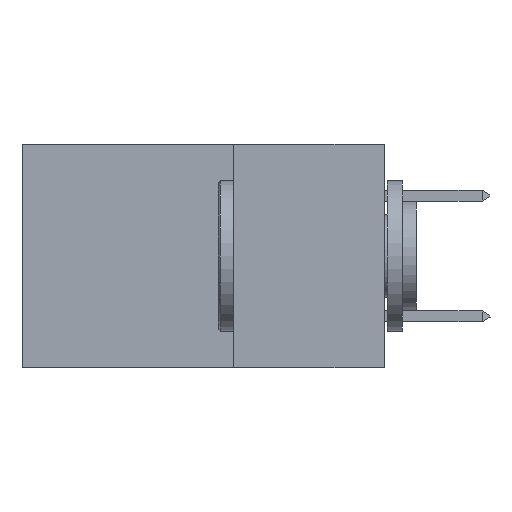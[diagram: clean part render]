
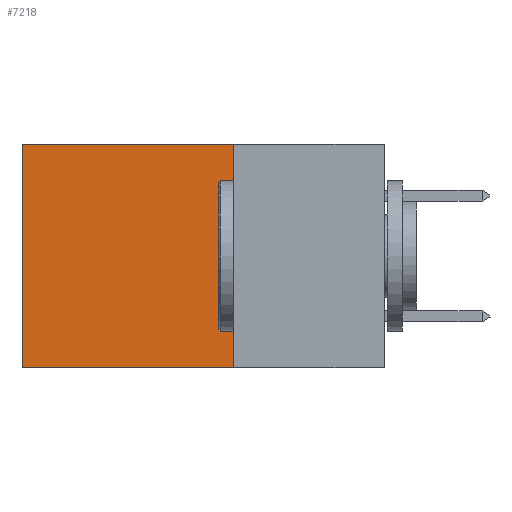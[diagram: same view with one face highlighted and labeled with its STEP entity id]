
A CAD part, left-side view. The second image highlights one B-rep face of the part: STEP entity #7218.
In plain terms, the highlighted planar face has unit normal (-1, 0, 0).
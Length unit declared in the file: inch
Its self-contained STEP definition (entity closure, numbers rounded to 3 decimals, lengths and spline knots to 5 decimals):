
#7 = FACE_OUTER_BOUND ( 'NONE', #13124, .T. ) ;
#71 = DIRECTION ( 'NONE',  ( 1., 0., 0. ) ) ;
#235 = CARTESIAN_POINT ( 'NONE',  ( 0.2875, 0.25, 0. ) ) ;
#415 = VECTOR ( 'NONE', #11790, 39.37008 ) ;
#1043 = ORIENTED_EDGE ( 'NONE', *, *, #7976, .F. ) ;
#1369 = EDGE_CURVE ( 'NONE', #7098, #1430, #12800, .T. ) ;
#1430 = VERTEX_POINT ( 'NONE', #6692 ) ;
#2300 = LINE ( 'NONE', #13733, #8791 ) ;
#2310 = VECTOR ( 'NONE', #9135, 39.37008 ) ;
#2949 = CARTESIAN_POINT ( 'NONE',  ( 0.2875, 0.25, -0.37 ) ) ;
#3578 = DIRECTION ( 'NONE',  ( 0., 1., 0. ) ) ;
#3686 = PLANE ( 'NONE',  #6498 ) ;
#3826 = CARTESIAN_POINT ( 'NONE',  ( 0.2875, 0.25, 0. ) ) ;
#4087 = LINE ( 'NONE', #6836, #2310 ) ;
#4740 = DIRECTION ( 'NONE',  ( 0., 1., 0. ) ) ;
#6018 = EDGE_CURVE ( 'NONE', #7098, #9518, #9941, .T. ) ;
#6498 = AXIS2_PLACEMENT_3D ( 'NONE', #235, #71, #8244 ) ;
#6692 = CARTESIAN_POINT ( 'NONE',  ( 0.2875, 0.6, 0. ) ) ;
#6818 = VERTEX_POINT ( 'NONE', #8140 ) ;
#6836 = CARTESIAN_POINT ( 'NONE',  ( 0.2875, 0.6, 0. ) ) ;
#7098 = VERTEX_POINT ( 'NONE', #10481 ) ;
#7218 = ADVANCED_FACE ( 'NONE', ( #7 ), #3686, .F. ) ;
#7976 = EDGE_CURVE ( 'NONE', #9518, #6818, #2300, .T. ) ;
#8140 = CARTESIAN_POINT ( 'NONE',  ( 0.2875, 0.6, -0.37 ) ) ;
#8244 = DIRECTION ( 'NONE',  ( 0., 0., -1. ) ) ;
#8563 = ORIENTED_EDGE ( 'NONE', *, *, #6018, .F. ) ;
#8639 = ORIENTED_EDGE ( 'NONE', *, *, #11719, .T. ) ;
#8791 = VECTOR ( 'NONE', #4740, 39.37008 ) ;
#9135 = DIRECTION ( 'NONE',  ( 0., 0., -1. ) ) ;
#9518 = VERTEX_POINT ( 'NONE', #2949 ) ;
#9557 = ORIENTED_EDGE ( 'NONE', *, *, #1369, .T. ) ;
#9586 = CARTESIAN_POINT ( 'NONE',  ( 0.2875, 0.25, 0. ) ) ;
#9737 = VECTOR ( 'NONE', #3578, 39.37008 ) ;
#9941 = LINE ( 'NONE', #3826, #415 ) ;
#10481 = CARTESIAN_POINT ( 'NONE',  ( 0.2875, 0.25, 0. ) ) ;
#11719 = EDGE_CURVE ( 'NONE', #1430, #6818, #4087, .T. ) ;
#11790 = DIRECTION ( 'NONE',  ( 0., 0., -1. ) ) ;
#12800 = LINE ( 'NONE', #9586, #9737 ) ;
#13124 = EDGE_LOOP ( 'NONE', ( #8639, #1043, #8563, #9557 ) ) ;
#13733 = CARTESIAN_POINT ( 'NONE',  ( 0.2875, 0.25, -0.37 ) ) ;
